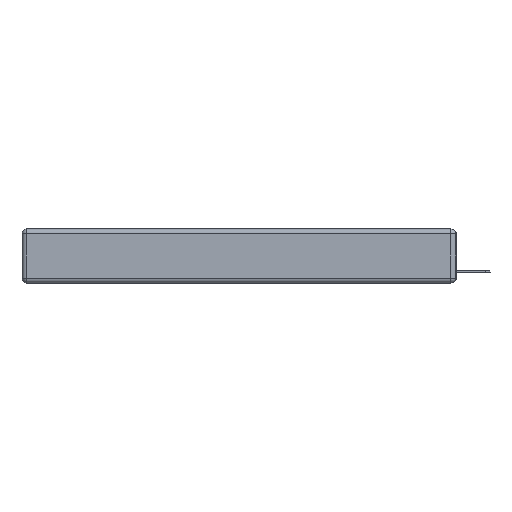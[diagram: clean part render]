
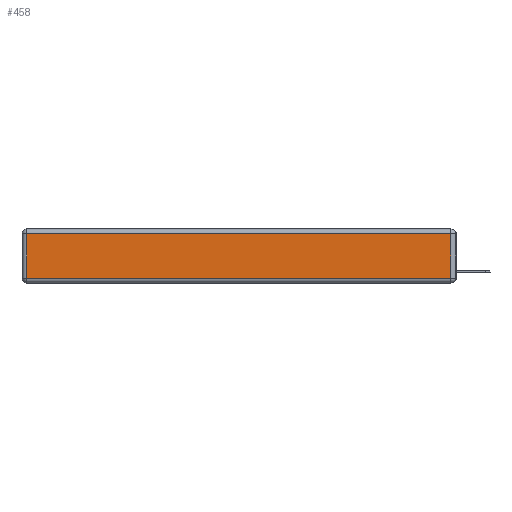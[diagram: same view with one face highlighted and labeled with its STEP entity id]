
A CAD part, left-side view. The second image highlights one B-rep face of the part: STEP entity #458.
In plain terms, the highlighted planar face has unit normal (-1, 0, 0).
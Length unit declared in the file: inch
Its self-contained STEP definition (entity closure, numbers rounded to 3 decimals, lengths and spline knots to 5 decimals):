
#25 = VECTOR ( 'NONE', #2597, 39.37008 ) ;
#106 = EDGE_CURVE ( 'NONE', #9836, #4727, #9141, .T. ) ;
#290 = ORIENTED_EDGE ( 'NONE', *, *, #8989, .T. ) ;
#376 = ORIENTED_EDGE ( 'NONE', *, *, #7853, .T. ) ;
#391 = LINE ( 'NONE', #4896, #25 ) ;
#458 = ADVANCED_FACE ( 'NONE', ( #9059 ), #5526, .T. ) ;
#1064 = LINE ( 'NONE', #2465, #11823 ) ;
#2465 = CARTESIAN_POINT ( 'NONE',  ( 0., 2.75, -0.03 ) ) ;
#2597 = DIRECTION ( 'NONE',  ( 0., -1., 0. ) ) ;
#3859 = EDGE_LOOP ( 'NONE', ( #12240, #14127, #290, #376 ) ) ;
#3919 = CARTESIAN_POINT ( 'NONE',  ( 0., 2.72, -0.343 ) ) ;
#4107 = CARTESIAN_POINT ( 'NONE',  ( 0., 0.03, -0.03 ) ) ;
#4550 = DIRECTION ( 'NONE',  ( 0., 0., 1. ) ) ;
#4694 = AXIS2_PLACEMENT_3D ( 'NONE', #11053, #6777, #4550 ) ;
#4727 = VERTEX_POINT ( 'NONE', #4107 ) ;
#4896 = CARTESIAN_POINT ( 'NONE',  ( 0., 0., -0.313 ) ) ;
#5023 = EDGE_CURVE ( 'NONE', #5766, #9836, #391, .T. ) ;
#5172 = VECTOR ( 'NONE', #12533, 39.37008 ) ;
#5526 = PLANE ( 'NONE',  #4694 ) ;
#5543 = CARTESIAN_POINT ( 'NONE',  ( 0., 0.03, -0.343 ) ) ;
#5766 = VERTEX_POINT ( 'NONE', #7639 ) ;
#5836 = VECTOR ( 'NONE', #8587, 39.37008 ) ;
#6777 = DIRECTION ( 'NONE',  ( -1., 0., 0. ) ) ;
#6852 = CARTESIAN_POINT ( 'NONE',  ( 0., 0.03, -0.313 ) ) ;
#7639 = CARTESIAN_POINT ( 'NONE',  ( 0., 2.72, -0.313 ) ) ;
#7853 = EDGE_CURVE ( 'NONE', #9091, #5766, #13996, .T. ) ;
#8587 = DIRECTION ( 'NONE',  ( 0., 0., -1. ) ) ;
#8588 = CARTESIAN_POINT ( 'NONE',  ( 0., 2.72, -0.03 ) ) ;
#8989 = EDGE_CURVE ( 'NONE', #4727, #9091, #1064, .T. ) ;
#9059 = FACE_OUTER_BOUND ( 'NONE', #3859, .T. ) ;
#9091 = VERTEX_POINT ( 'NONE', #8588 ) ;
#9141 = LINE ( 'NONE', #5543, #5172 ) ;
#9836 = VERTEX_POINT ( 'NONE', #6852 ) ;
#11053 = CARTESIAN_POINT ( 'NONE',  ( 0., 0., -0.343 ) ) ;
#11324 = DIRECTION ( 'NONE',  ( 0., 1., 0. ) ) ;
#11823 = VECTOR ( 'NONE', #11324, 39.37008 ) ;
#12240 = ORIENTED_EDGE ( 'NONE', *, *, #5023, .T. ) ;
#12533 = DIRECTION ( 'NONE',  ( 0., 0., 1. ) ) ;
#13996 = LINE ( 'NONE', #3919, #5836 ) ;
#14127 = ORIENTED_EDGE ( 'NONE', *, *, #106, .T. ) ;
